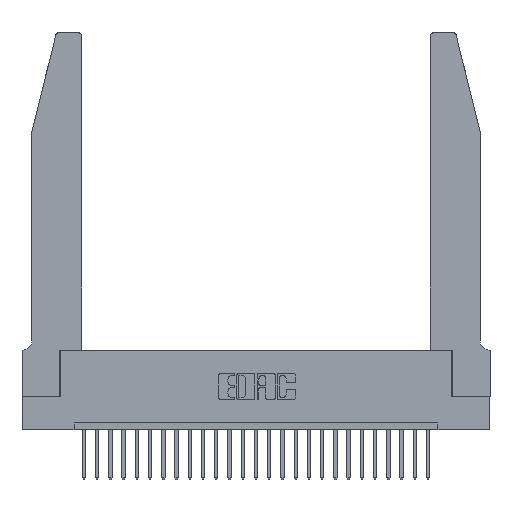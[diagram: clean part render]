
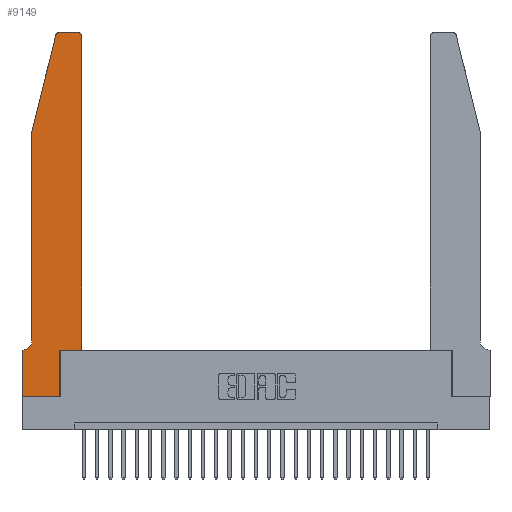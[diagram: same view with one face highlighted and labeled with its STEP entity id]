
A CAD part, top view. The second image highlights one B-rep face of the part: STEP entity #9149.
In plain terms, the highlighted planar face has unit normal (0, 0, 1).
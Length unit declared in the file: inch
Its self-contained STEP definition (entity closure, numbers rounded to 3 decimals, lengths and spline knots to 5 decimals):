
#201 = EDGE_CURVE ( 'NONE', #9403, #14101, #2375, .T. ) ;
#249 = LINE ( 'NONE', #1793, #8466 ) ;
#278 = CARTESIAN_POINT ( 'NONE',  ( 0.2865, 0., 0.37 ) ) ;
#387 = ORIENTED_EDGE ( 'NONE', *, *, #23089, .T. ) ;
#446 = DIRECTION ( 'NONE',  ( 0., -1., 0. ) ) ;
#1498 = ORIENTED_EDGE ( 'NONE', *, *, #22979, .T. ) ;
#1793 = CARTESIAN_POINT ( 'NONE',  ( 0.0755, 0.35, 0.37 ) ) ;
#2097 = VERTEX_POINT ( 'NONE', #14578 ) ;
#2278 = DIRECTION ( 'NONE',  ( 0., 1., 0. ) ) ;
#2375 = LINE ( 'NONE', #6215, #20397 ) ;
#2436 = CARTESIAN_POINT ( 'NONE',  ( 0.0055, 0.35, 0.37 ) ) ;
#2669 = CARTESIAN_POINT ( 'NONE',  ( 0.284, 2.72, 0.37 ) ) ;
#2731 = CIRCLE ( 'NONE', #26144, 0.03 ) ;
#2842 = DIRECTION ( 'NONE',  ( 1., 0., 0. ) ) ;
#2903 = EDGE_CURVE ( 'NONE', #2097, #6245, #16978, .T. ) ;
#2961 = ORIENTED_EDGE ( 'NONE', *, *, #26915, .T. ) ;
#3352 = EDGE_CURVE ( 'NONE', #6245, #21159, #249, .T. ) ;
#3424 = DIRECTION ( 'NONE',  ( 0., 1., 0. ) ) ;
#3935 = DIRECTION ( 'NONE',  ( -1., 0., 0. ) ) ;
#3938 = CARTESIAN_POINT ( 'NONE',  ( 0.0055, 0.42, 0.37 ) ) ;
#4135 = EDGE_CURVE ( 'NONE', #14101, #2097, #23420, .T. ) ;
#4811 = AXIS2_PLACEMENT_3D ( 'NONE', #10124, #24522, #9775 ) ;
#4866 = CARTESIAN_POINT ( 'NONE',  ( 0.2605, 2.75, 0.37 ) ) ;
#4951 = ORIENTED_EDGE ( 'NONE', *, *, #10140, .T. ) ;
#5501 = VERTEX_POINT ( 'NONE', #22917 ) ;
#5539 = CARTESIAN_POINT ( 'NONE',  ( 0.4505, 0.35, 0.37 ) ) ;
#5809 = VECTOR ( 'NONE', #24262, 39.37008 ) ;
#5956 = DIRECTION ( 'NONE',  ( -0.239, -0.971, 0. ) ) ;
#6106 = DIRECTION ( 'NONE',  ( -1., 0., 0. ) ) ;
#6146 = VERTEX_POINT ( 'NONE', #278 ) ;
#6215 = CARTESIAN_POINT ( 'NONE',  ( 0.0755, 2., 0.37 ) ) ;
#6245 = VERTEX_POINT ( 'NONE', #2436 ) ;
#6464 = CARTESIAN_POINT ( 'NONE',  ( 0.25487, 2.72718, 0.37 ) ) ;
#6849 = CARTESIAN_POINT ( 'NONE',  ( 0., 0., 0.37 ) ) ;
#7113 = DIRECTION ( 'NONE',  ( 1., 0., 0. ) ) ;
#7439 = CARTESIAN_POINT ( 'NONE',  ( 0.4505, 0.35, 0.37 ) ) ;
#7725 = CARTESIAN_POINT ( 'NONE',  ( 0.4205, 2.72, 0.37 ) ) ;
#8057 = PLANE ( 'NONE',  #4811 ) ;
#8303 = ORIENTED_EDGE ( 'NONE', *, *, #3352, .T. ) ;
#8466 = VECTOR ( 'NONE', #3935, 39.37008 ) ;
#9149 = ADVANCED_FACE ( 'NONE', ( #20873 ), #8057, .T. ) ;
#9403 = VERTEX_POINT ( 'NONE', #6464 ) ;
#9775 = DIRECTION ( 'NONE',  ( 1., 0., 0. ) ) ;
#10124 = CARTESIAN_POINT ( 'NONE',  ( 0., 0.35, 0.37 ) ) ;
#10140 = EDGE_CURVE ( 'NONE', #10569, #22309, #21829, .T. ) ;
#10412 = VECTOR ( 'NONE', #3424, 39.37008 ) ;
#10569 = VERTEX_POINT ( 'NONE', #23845 ) ;
#10709 = ORIENTED_EDGE ( 'NONE', *, *, #201, .T. ) ;
#10943 = VECTOR ( 'NONE', #446, 39.37008 ) ;
#10964 = VECTOR ( 'NONE', #7113, 39.37008 ) ;
#11386 = AXIS2_PLACEMENT_3D ( 'NONE', #3938, #12395, #6106 ) ;
#11609 = LINE ( 'NONE', #6849, #10943 ) ;
#11997 = CARTESIAN_POINT ( 'NONE',  ( 0.4505, 0.35, 0.37 ) ) ;
#12087 = ORIENTED_EDGE ( 'NONE', *, *, #4135, .T. ) ;
#12395 = DIRECTION ( 'NONE',  ( 0., 0., -1. ) ) ;
#12494 = CARTESIAN_POINT ( 'NONE',  ( 0.0755, 2., 0.37 ) ) ;
#12947 = CARTESIAN_POINT ( 'NONE',  ( 0.2865, 0.35, 0.37 ) ) ;
#13717 = EDGE_LOOP ( 'NONE', ( #1498, #25650, #10709, #12087, #23428, #8303, #23044, #18554, #18521, #4951, #2961, #387 ) ) ;
#14021 = LINE ( 'NONE', #4866, #17995 ) ;
#14101 = VERTEX_POINT ( 'NONE', #12494 ) ;
#14245 = LINE ( 'NONE', #15013, #10964 ) ;
#14578 = CARTESIAN_POINT ( 'NONE',  ( 0.0755, 0.42, 0.37 ) ) ;
#15013 = CARTESIAN_POINT ( 'NONE',  ( 0., 0., 0.37 ) ) ;
#15291 = EDGE_CURVE ( 'NONE', #19718, #6146, #14245, .T. ) ;
#15449 = CARTESIAN_POINT ( 'NONE',  ( 0.4205, 2.75, 0.37 ) ) ;
#16255 = EDGE_CURVE ( 'NONE', #5501, #9403, #2731, .T. ) ;
#16615 = DIRECTION ( 'NONE',  ( 0., -1., 0. ) ) ;
#16978 = CIRCLE ( 'NONE', #11386, 0.07 ) ;
#16980 = LINE ( 'NONE', #12947, #17199 ) ;
#17199 = VECTOR ( 'NONE', #2278, 39.37008 ) ;
#17313 = DIRECTION ( 'NONE',  ( -1., 0., 0. ) ) ;
#17995 = VECTOR ( 'NONE', #17313, 39.37008 ) ;
#18210 = VECTOR ( 'NONE', #16615, 39.37008 ) ;
#18309 = DIRECTION ( 'NONE',  ( 0., 0., 1. ) ) ;
#18405 = DIRECTION ( 'NONE',  ( 1., 0., 0. ) ) ;
#18521 = ORIENTED_EDGE ( 'NONE', *, *, #23374, .T. ) ;
#18554 = ORIENTED_EDGE ( 'NONE', *, *, #15291, .T. ) ;
#18752 = VERTEX_POINT ( 'NONE', #15449 ) ;
#19582 = DIRECTION ( 'NONE',  ( 0., 0., 1. ) ) ;
#19718 = VERTEX_POINT ( 'NONE', #22470 ) ;
#19947 = CIRCLE ( 'NONE', #26275, 0.03 ) ;
#20234 = LINE ( 'NONE', #11997, #10412 ) ;
#20397 = VECTOR ( 'NONE', #5956, 39.37008 ) ;
#20416 = EDGE_CURVE ( 'NONE', #21159, #19718, #11609, .T. ) ;
#20873 = FACE_OUTER_BOUND ( 'NONE', #13717, .T. ) ;
#21159 = VERTEX_POINT ( 'NONE', #23025 ) ;
#21829 = LINE ( 'NONE', #7439, #5809 ) ;
#22309 = VERTEX_POINT ( 'NONE', #5539 ) ;
#22470 = CARTESIAN_POINT ( 'NONE',  ( 0., 0., 0.37 ) ) ;
#22643 = CARTESIAN_POINT ( 'NONE',  ( 0.0755, 2., 0.37 ) ) ;
#22917 = CARTESIAN_POINT ( 'NONE',  ( 0.284, 2.75, 0.37 ) ) ;
#22979 = EDGE_CURVE ( 'NONE', #18752, #5501, #14021, .T. ) ;
#23025 = CARTESIAN_POINT ( 'NONE',  ( 0., 0.35, 0.37 ) ) ;
#23044 = ORIENTED_EDGE ( 'NONE', *, *, #20416, .T. ) ;
#23089 = EDGE_CURVE ( 'NONE', #23434, #18752, #19947, .T. ) ;
#23374 = EDGE_CURVE ( 'NONE', #6146, #10569, #16980, .T. ) ;
#23420 = LINE ( 'NONE', #22643, #18210 ) ;
#23428 = ORIENTED_EDGE ( 'NONE', *, *, #2903, .T. ) ;
#23434 = VERTEX_POINT ( 'NONE', #25809 ) ;
#23845 = CARTESIAN_POINT ( 'NONE',  ( 0.2865, 0.35, 0.37 ) ) ;
#24262 = DIRECTION ( 'NONE',  ( 1., 0., 0. ) ) ;
#24522 = DIRECTION ( 'NONE',  ( 0., 0., 1. ) ) ;
#25650 = ORIENTED_EDGE ( 'NONE', *, *, #16255, .T. ) ;
#25809 = CARTESIAN_POINT ( 'NONE',  ( 0.4505, 2.72, 0.37 ) ) ;
#26144 = AXIS2_PLACEMENT_3D ( 'NONE', #2669, #19582, #2842 ) ;
#26275 = AXIS2_PLACEMENT_3D ( 'NONE', #7725, #18309, #18405 ) ;
#26915 = EDGE_CURVE ( 'NONE', #22309, #23434, #20234, .T. ) ;
